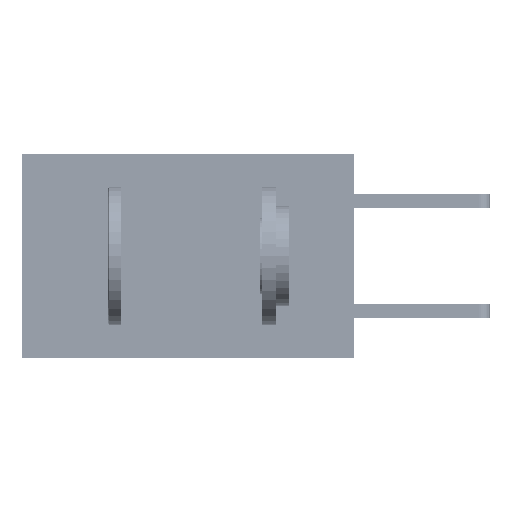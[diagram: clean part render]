
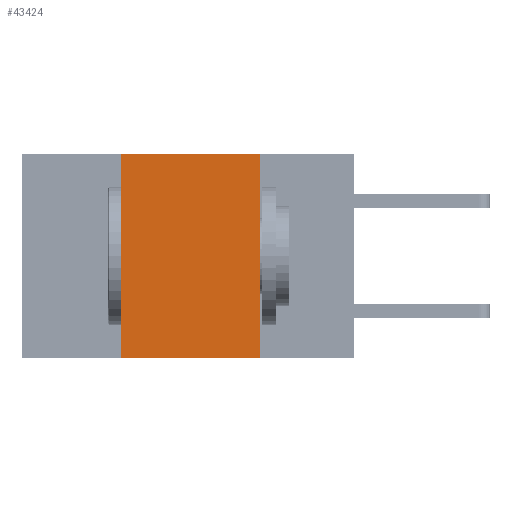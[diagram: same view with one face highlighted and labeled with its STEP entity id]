
A CAD part, left-side view. The second image highlights one B-rep face of the part: STEP entity #43424.
In plain terms, the highlighted planar face has unit normal (-1, 0, 0).
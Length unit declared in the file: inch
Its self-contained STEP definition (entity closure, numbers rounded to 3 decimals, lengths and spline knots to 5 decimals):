
#359 = CARTESIAN_POINT ( 'NONE',  ( 0., 0.6, 0. ) ) ;
#1367 = VECTOR ( 'NONE', #14999, 39.37008 ) ;
#5015 = VECTOR ( 'NONE', #26413, 39.37008 ) ;
#7166 = LINE ( 'NONE', #35838, #5015 ) ;
#10003 = LINE ( 'NONE', #21343, #1367 ) ;
#11075 = EDGE_CURVE ( 'NONE', #36025, #20470, #29847, .T. ) ;
#14494 = DIRECTION ( 'NONE',  ( 1., 0., 0. ) ) ;
#14547 = ORIENTED_EDGE ( 'NONE', *, *, #37934, .F. ) ;
#14999 = DIRECTION ( 'NONE',  ( 0., -1., 0. ) ) ;
#16592 = FACE_OUTER_BOUND ( 'NONE', #37704, .T. ) ;
#17524 = DIRECTION ( 'NONE',  ( 0., -1., 0. ) ) ;
#17782 = AXIS2_PLACEMENT_3D ( 'NONE', #41914, #14494, #35063 ) ;
#17809 = CARTESIAN_POINT ( 'NONE',  ( 0., 0.42, -0.37 ) ) ;
#20470 = VERTEX_POINT ( 'NONE', #43285 ) ;
#21343 = CARTESIAN_POINT ( 'NONE',  ( 0., 0.6, -0.37 ) ) ;
#21578 = PLANE ( 'NONE',  #17782 ) ;
#26413 = DIRECTION ( 'NONE',  ( 0., 0., -1. ) ) ;
#26794 = VECTOR ( 'NONE', #17524, 39.37008 ) ;
#27059 = EDGE_CURVE ( 'NONE', #40462, #30130, #7166, .T. ) ;
#29847 = LINE ( 'NONE', #34647, #36904 ) ;
#30130 = VERTEX_POINT ( 'NONE', #35022 ) ;
#30895 = DIRECTION ( 'NONE',  ( 0., 0., 1. ) ) ;
#34253 = ORIENTED_EDGE ( 'NONE', *, *, #27059, .F. ) ;
#34647 = CARTESIAN_POINT ( 'NONE',  ( 0., 0.42, 0. ) ) ;
#35022 = CARTESIAN_POINT ( 'NONE',  ( 0., 0.17, -0.37 ) ) ;
#35063 = DIRECTION ( 'NONE',  ( 0., 0., -1. ) ) ;
#35838 = CARTESIAN_POINT ( 'NONE',  ( 0., 0.17, 0. ) ) ;
#36025 = VERTEX_POINT ( 'NONE', #17809 ) ;
#36904 = VECTOR ( 'NONE', #30895, 39.37008 ) ;
#37132 = LINE ( 'NONE', #359, #26794 ) ;
#37704 = EDGE_LOOP ( 'NONE', ( #34253, #14547, #43180, #39608 ) ) ;
#37934 = EDGE_CURVE ( 'NONE', #20470, #40462, #37132, .T. ) ;
#39608 = ORIENTED_EDGE ( 'NONE', *, *, #44672, .T. ) ;
#40462 = VERTEX_POINT ( 'NONE', #41727 ) ;
#41727 = CARTESIAN_POINT ( 'NONE',  ( 0., 0.17, 0. ) ) ;
#41914 = CARTESIAN_POINT ( 'NONE',  ( 0., 0.6, 0. ) ) ;
#43180 = ORIENTED_EDGE ( 'NONE', *, *, #11075, .F. ) ;
#43285 = CARTESIAN_POINT ( 'NONE',  ( 0., 0.42, 0. ) ) ;
#43424 = ADVANCED_FACE ( 'NONE', ( #16592 ), #21578, .F. ) ;
#44672 = EDGE_CURVE ( 'NONE', #36025, #30130, #10003, .T. ) ;
